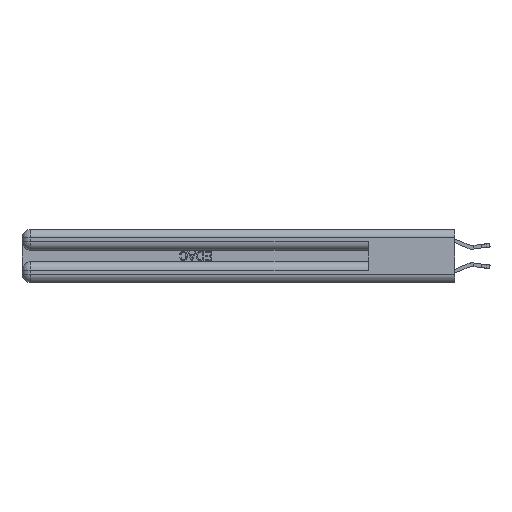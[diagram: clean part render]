
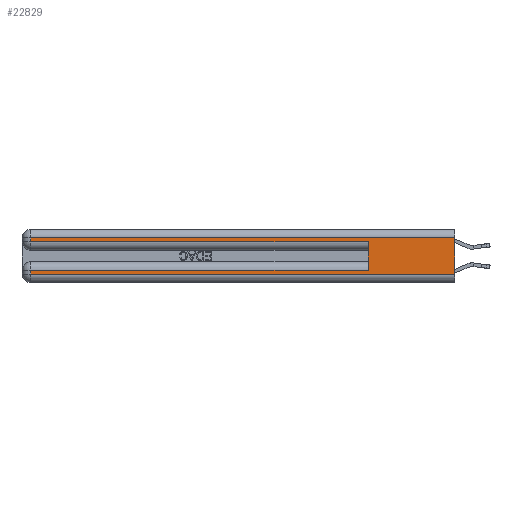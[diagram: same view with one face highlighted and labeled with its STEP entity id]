
A CAD part, left-side view. The second image highlights one B-rep face of the part: STEP entity #22829.
In plain terms, the highlighted planar face has unit normal (-1, 0, 0).
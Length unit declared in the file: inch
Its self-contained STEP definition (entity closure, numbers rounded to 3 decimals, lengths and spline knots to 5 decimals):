
#92 = DIRECTION ( 'NONE',  ( 0., 1., 0. ) ) ;
#382 = DIRECTION ( 'NONE',  ( 1., 0., 0. ) ) ;
#895 = ORIENTED_EDGE ( 'NONE', *, *, #27254, .F. ) ;
#1272 = LINE ( 'NONE', #30897, #29215 ) ;
#2162 = VECTOR ( 'NONE', #25912, 39.37008 ) ;
#2164 = CARTESIAN_POINT ( 'NONE',  ( 0., 0., 0.31 ) ) ;
#2926 = DIRECTION ( 'NONE',  ( 0., -1., 0. ) ) ;
#3988 = CARTESIAN_POINT ( 'NONE',  ( 0., 2.94, 0.37 ) ) ;
#4136 = LINE ( 'NONE', #3988, #29738 ) ;
#4509 = AXIS2_PLACEMENT_3D ( 'NONE', #26884, #382, #7536 ) ;
#4992 = LINE ( 'NONE', #24497, #10141 ) ;
#5209 = LINE ( 'NONE', #14742, #9936 ) ;
#5357 = CARTESIAN_POINT ( 'NONE',  ( 0., 0., 0.31 ) ) ;
#6401 = LINE ( 'NONE', #21003, #2162 ) ;
#7536 = DIRECTION ( 'NONE',  ( 0., 0., -1. ) ) ;
#7854 = ORIENTED_EDGE ( 'NONE', *, *, #8861, .T. ) ;
#8406 = CARTESIAN_POINT ( 'NONE',  ( 0., 2.94, 0.06 ) ) ;
#8861 = EDGE_CURVE ( 'NONE', #13786, #18954, #4136, .T. ) ;
#8977 = EDGE_CURVE ( 'NONE', #20360, #27190, #1272, .T. ) ;
#9293 = ORIENTED_EDGE ( 'NONE', *, *, #15265, .T. ) ;
#9936 = VECTOR ( 'NONE', #17772, 39.37008 ) ;
#10141 = VECTOR ( 'NONE', #2926, 39.37008 ) ;
#10861 = CARTESIAN_POINT ( 'NONE',  ( 0., 0., 0.06 ) ) ;
#10934 = VECTOR ( 'NONE', #30107, 39.37008 ) ;
#11544 = VERTEX_POINT ( 'NONE', #10861 ) ;
#12188 = VERTEX_POINT ( 'NONE', #5357 ) ;
#13786 = VERTEX_POINT ( 'NONE', #16815 ) ;
#14742 = CARTESIAN_POINT ( 'NONE',  ( 0., 2.94, 0.37 ) ) ;
#15008 = EDGE_CURVE ( 'NONE', #12188, #11544, #16197, .T. ) ;
#15265 = EDGE_CURVE ( 'NONE', #27190, #23935, #5209, .T. ) ;
#15451 = CARTESIAN_POINT ( 'NONE',  ( 0., 0., 0.285 ) ) ;
#15996 = VECTOR ( 'NONE', #17697, 39.37008 ) ;
#16197 = LINE ( 'NONE', #25865, #10934 ) ;
#16277 = EDGE_CURVE ( 'NONE', #18954, #17981, #18164, .T. ) ;
#16616 = ORIENTED_EDGE ( 'NONE', *, *, #29905, .T. ) ;
#16815 = CARTESIAN_POINT ( 'NONE',  ( 0., 2.94, 0.31 ) ) ;
#17386 = CARTESIAN_POINT ( 'NONE',  ( 0., 0.6, 0.285 ) ) ;
#17697 = DIRECTION ( 'NONE',  ( 0., -1., 0. ) ) ;
#17772 = DIRECTION ( 'NONE',  ( 0., 0., -1. ) ) ;
#17902 = EDGE_LOOP ( 'NONE', ( #18190, #16616, #7854, #23146, #895, #23289, #9293, #19865 ) ) ;
#17981 = VERTEX_POINT ( 'NONE', #17386 ) ;
#18164 = LINE ( 'NONE', #15451, #15996 ) ;
#18190 = ORIENTED_EDGE ( 'NONE', *, *, #15008, .F. ) ;
#18954 = VERTEX_POINT ( 'NONE', #25495 ) ;
#19441 = PLANE ( 'NONE',  #4509 ) ;
#19865 = ORIENTED_EDGE ( 'NONE', *, *, #21614, .T. ) ;
#20360 = VERTEX_POINT ( 'NONE', #27670 ) ;
#21003 = CARTESIAN_POINT ( 'NONE',  ( 0., 0.6, 0.145 ) ) ;
#21028 = VECTOR ( 'NONE', #92, 39.37008 ) ;
#21614 = EDGE_CURVE ( 'NONE', #23935, #11544, #4992, .T. ) ;
#22829 = ADVANCED_FACE ( 'NONE', ( #29235 ), #19441, .F. ) ;
#23146 = ORIENTED_EDGE ( 'NONE', *, *, #16277, .T. ) ;
#23289 = ORIENTED_EDGE ( 'NONE', *, *, #8977, .T. ) ;
#23537 = CARTESIAN_POINT ( 'NONE',  ( 0., 2.94, 0.085 ) ) ;
#23935 = VERTEX_POINT ( 'NONE', #8406 ) ;
#24110 = DIRECTION ( 'NONE',  ( 0., 1., 0. ) ) ;
#24497 = CARTESIAN_POINT ( 'NONE',  ( 0., 0., 0.06 ) ) ;
#25400 = DIRECTION ( 'NONE',  ( 0., 0., -1. ) ) ;
#25495 = CARTESIAN_POINT ( 'NONE',  ( 0., 2.94, 0.285 ) ) ;
#25865 = CARTESIAN_POINT ( 'NONE',  ( 0., 0., 0.37 ) ) ;
#25912 = DIRECTION ( 'NONE',  ( 0., 0., 1. ) ) ;
#26884 = CARTESIAN_POINT ( 'NONE',  ( 0., 0., 0.37 ) ) ;
#27190 = VERTEX_POINT ( 'NONE', #23537 ) ;
#27254 = EDGE_CURVE ( 'NONE', #20360, #17981, #6401, .T. ) ;
#27670 = CARTESIAN_POINT ( 'NONE',  ( 0., 0.6, 0.085 ) ) ;
#29215 = VECTOR ( 'NONE', #24110, 39.37008 ) ;
#29235 = FACE_OUTER_BOUND ( 'NONE', #17902, .T. ) ;
#29738 = VECTOR ( 'NONE', #25400, 39.37008 ) ;
#29905 = EDGE_CURVE ( 'NONE', #12188, #13786, #31162, .T. ) ;
#30107 = DIRECTION ( 'NONE',  ( 0., 0., -1. ) ) ;
#30897 = CARTESIAN_POINT ( 'NONE',  ( 0., 0., 0.085 ) ) ;
#31162 = LINE ( 'NONE', #2164, #21028 ) ;
